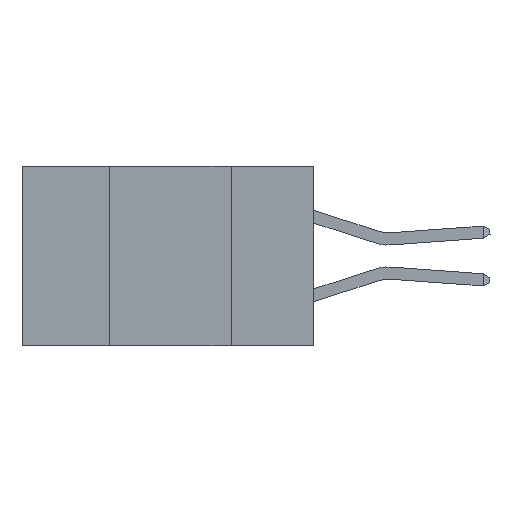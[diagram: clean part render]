
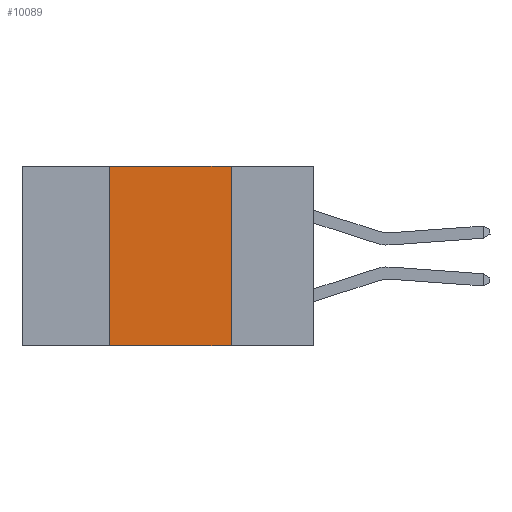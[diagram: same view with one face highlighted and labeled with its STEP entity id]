
A CAD part, left-side view. The second image highlights one B-rep face of the part: STEP entity #10089.
In plain terms, the highlighted planar face has unit normal (-1, 0, 0).
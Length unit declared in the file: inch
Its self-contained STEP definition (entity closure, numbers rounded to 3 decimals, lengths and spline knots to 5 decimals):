
#286 = VERTEX_POINT ( 'NONE', #22351 ) ;
#337 = ORIENTED_EDGE ( 'NONE', *, *, #18910, .F. ) ;
#600 = LINE ( 'NONE', #19558, #9033 ) ;
#1519 = DIRECTION ( 'NONE',  ( 0., 0., -1. ) ) ;
#2199 = CARTESIAN_POINT ( 'NONE',  ( 0., 0.6, 0. ) ) ;
#2687 = EDGE_CURVE ( 'NONE', #286, #4318, #4950, .T. ) ;
#3501 = CARTESIAN_POINT ( 'NONE',  ( 0., 0.17, -0.37 ) ) ;
#3824 = DIRECTION ( 'NONE',  ( 0., 0., -1. ) ) ;
#3914 = PLANE ( 'NONE',  #23563 ) ;
#3967 = CARTESIAN_POINT ( 'NONE',  ( 0., 0.42, -0.37 ) ) ;
#4318 = VERTEX_POINT ( 'NONE', #3501 ) ;
#4402 = FACE_OUTER_BOUND ( 'NONE', #7804, .T. ) ;
#4809 = VECTOR ( 'NONE', #13630, 39.37008 ) ;
#4950 = LINE ( 'NONE', #22056, #22657 ) ;
#5220 = EDGE_CURVE ( 'NONE', #8032, #286, #14974, .T. ) ;
#5387 = LINE ( 'NONE', #16938, #14688 ) ;
#7571 = CARTESIAN_POINT ( 'NONE',  ( 0., 0.42, 0. ) ) ;
#7804 = EDGE_LOOP ( 'NONE', ( #17463, #8292, #337, #16293 ) ) ;
#8032 = VERTEX_POINT ( 'NONE', #7571 ) ;
#8292 = ORIENTED_EDGE ( 'NONE', *, *, #5220, .F. ) ;
#9033 = VECTOR ( 'NONE', #10275, 39.37008 ) ;
#10089 = ADVANCED_FACE ( 'NONE', ( #4402 ), #3914, .F. ) ;
#10275 = DIRECTION ( 'NONE',  ( 0., -1., 0. ) ) ;
#13224 = DIRECTION ( 'NONE',  ( 0., 0., 1. ) ) ;
#13431 = DIRECTION ( 'NONE',  ( 1., 0., 0. ) ) ;
#13468 = CARTESIAN_POINT ( 'NONE',  ( 0., 0.6, 0. ) ) ;
#13630 = DIRECTION ( 'NONE',  ( 0., -1., 0. ) ) ;
#14688 = VECTOR ( 'NONE', #13224, 39.37008 ) ;
#14974 = LINE ( 'NONE', #13468, #4809 ) ;
#15561 = VERTEX_POINT ( 'NONE', #3967 ) ;
#16293 = ORIENTED_EDGE ( 'NONE', *, *, #21130, .T. ) ;
#16938 = CARTESIAN_POINT ( 'NONE',  ( 0., 0.42, 0. ) ) ;
#17463 = ORIENTED_EDGE ( 'NONE', *, *, #2687, .F. ) ;
#18910 = EDGE_CURVE ( 'NONE', #15561, #8032, #5387, .T. ) ;
#19558 = CARTESIAN_POINT ( 'NONE',  ( 0., 0.6, -0.37 ) ) ;
#21130 = EDGE_CURVE ( 'NONE', #15561, #4318, #600, .T. ) ;
#22056 = CARTESIAN_POINT ( 'NONE',  ( 0., 0.17, 0. ) ) ;
#22351 = CARTESIAN_POINT ( 'NONE',  ( 0., 0.17, 0. ) ) ;
#22657 = VECTOR ( 'NONE', #1519, 39.37008 ) ;
#23563 = AXIS2_PLACEMENT_3D ( 'NONE', #2199, #13431, #3824 ) ;
